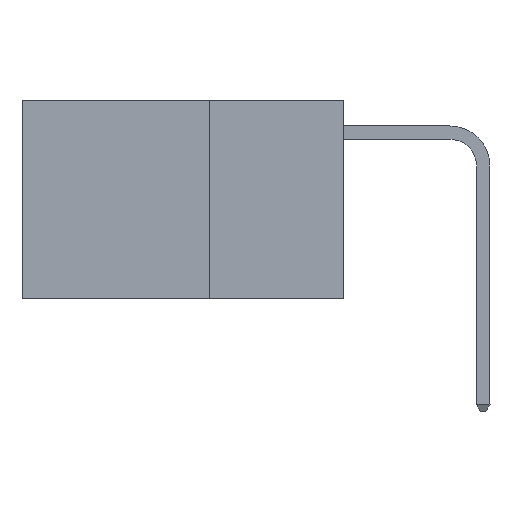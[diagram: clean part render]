
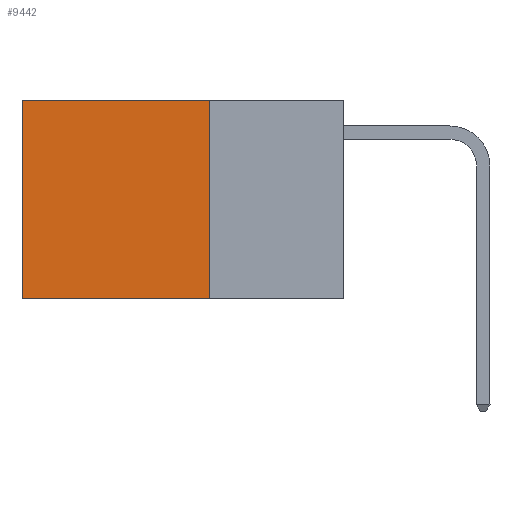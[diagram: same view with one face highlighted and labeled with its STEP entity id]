
A CAD part, left-side view. The second image highlights one B-rep face of the part: STEP entity #9442.
In plain terms, the highlighted planar face has unit normal (-1, 0, 0).
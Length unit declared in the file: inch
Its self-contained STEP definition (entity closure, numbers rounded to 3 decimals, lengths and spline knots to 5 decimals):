
#224 = VECTOR ( 'NONE', #5058, 39.37008 ) ;
#503 = DIRECTION ( 'NONE',  ( 0., 1., 0. ) ) ;
#550 = CARTESIAN_POINT ( 'NONE',  ( 0.2625, 0.25, 0. ) ) ;
#599 = EDGE_CURVE ( 'NONE', #7952, #9215, #5794, .T. ) ;
#791 = LINE ( 'NONE', #550, #5031 ) ;
#1305 = EDGE_CURVE ( 'NONE', #5310, #9025, #1908, .T. ) ;
#1908 = LINE ( 'NONE', #9009, #8757 ) ;
#2189 = CARTESIAN_POINT ( 'NONE',  ( 0.2625, 0.25, 0. ) ) ;
#2305 = CARTESIAN_POINT ( 'NONE',  ( 0.2625, 0.25, 0. ) ) ;
#2624 = LINE ( 'NONE', #5039, #224 ) ;
#3200 = DIRECTION ( 'NONE',  ( 0., 0., -1. ) ) ;
#4080 = PLANE ( 'NONE',  #11269 ) ;
#4598 = CARTESIAN_POINT ( 'NONE',  ( 0.2625, 0.6, -0.37 ) ) ;
#4613 = ORIENTED_EDGE ( 'NONE', *, *, #599, .T. ) ;
#4783 = ORIENTED_EDGE ( 'NONE', *, *, #6063, .F. ) ;
#4869 = DIRECTION ( 'NONE',  ( 0., 0., -1. ) ) ;
#5031 = VECTOR ( 'NONE', #503, 39.37008 ) ;
#5039 = CARTESIAN_POINT ( 'NONE',  ( 0.2625, 0.25, -0.37 ) ) ;
#5058 = DIRECTION ( 'NONE',  ( 0., 1., 0. ) ) ;
#5310 = VERTEX_POINT ( 'NONE', #2189 ) ;
#5481 = VECTOR ( 'NONE', #4869, 39.37008 ) ;
#5631 = EDGE_CURVE ( 'NONE', #5310, #7952, #791, .T. ) ;
#5794 = LINE ( 'NONE', #7420, #5481 ) ;
#6006 = EDGE_LOOP ( 'NONE', ( #4613, #4783, #7028, #7044 ) ) ;
#6063 = EDGE_CURVE ( 'NONE', #9025, #9215, #2624, .T. ) ;
#6304 = FACE_OUTER_BOUND ( 'NONE', #6006, .T. ) ;
#7028 = ORIENTED_EDGE ( 'NONE', *, *, #1305, .F. ) ;
#7044 = ORIENTED_EDGE ( 'NONE', *, *, #5631, .T. ) ;
#7420 = CARTESIAN_POINT ( 'NONE',  ( 0.2625, 0.6, 0. ) ) ;
#7952 = VERTEX_POINT ( 'NONE', #7972 ) ;
#7972 = CARTESIAN_POINT ( 'NONE',  ( 0.2625, 0.6, 0. ) ) ;
#8571 = DIRECTION ( 'NONE',  ( 1., 0., 0. ) ) ;
#8757 = VECTOR ( 'NONE', #11176, 39.37008 ) ;
#9009 = CARTESIAN_POINT ( 'NONE',  ( 0.2625, 0.25, 0. ) ) ;
#9025 = VERTEX_POINT ( 'NONE', #11331 ) ;
#9215 = VERTEX_POINT ( 'NONE', #4598 ) ;
#9442 = ADVANCED_FACE ( 'NONE', ( #6304 ), #4080, .F. ) ;
#11176 = DIRECTION ( 'NONE',  ( 0., 0., -1. ) ) ;
#11269 = AXIS2_PLACEMENT_3D ( 'NONE', #2305, #8571, #3200 ) ;
#11331 = CARTESIAN_POINT ( 'NONE',  ( 0.2625, 0.25, -0.37 ) ) ;
